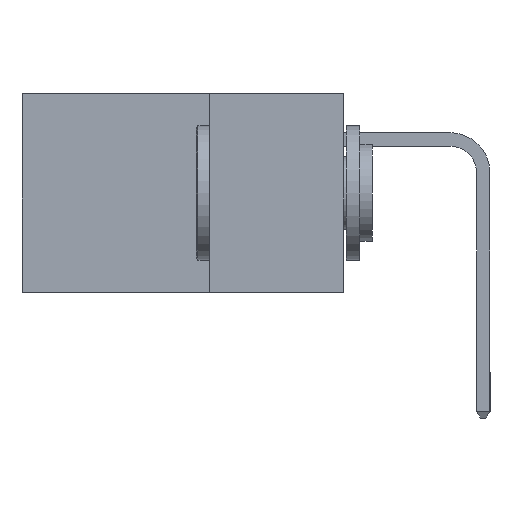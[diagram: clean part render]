
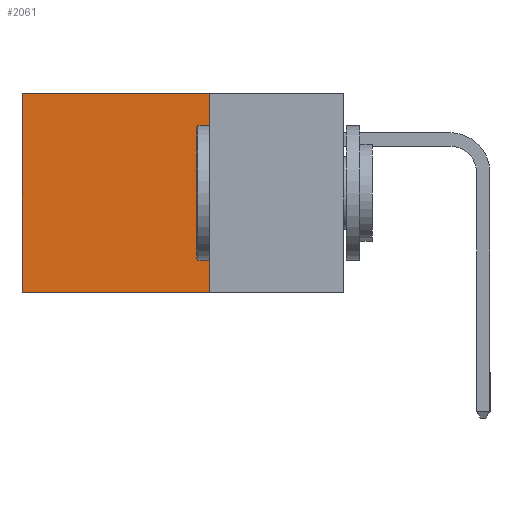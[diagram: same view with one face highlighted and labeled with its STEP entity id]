
A CAD part, left-side view. The second image highlights one B-rep face of the part: STEP entity #2061.
In plain terms, the highlighted planar face has unit normal (-1, 0, 0).
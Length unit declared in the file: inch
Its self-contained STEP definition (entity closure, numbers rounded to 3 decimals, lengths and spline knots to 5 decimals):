
#378 = DIRECTION ( 'NONE',  ( 0., 0., -1. ) ) ;
#1413 = VECTOR ( 'NONE', #378, 39.37008 ) ;
#1704 = CARTESIAN_POINT ( 'NONE',  ( 0.2615, 0.6, -0.37 ) ) ;
#2061 = ADVANCED_FACE ( 'NONE', ( #18170 ), #12680, .F. ) ;
#2657 = VECTOR ( 'NONE', #5814, 39.37008 ) ;
#2699 = LINE ( 'NONE', #21167, #17627 ) ;
#3039 = CARTESIAN_POINT ( 'NONE',  ( 0.2615, 0.25, -0.37 ) ) ;
#4036 = VECTOR ( 'NONE', #19796, 39.37008 ) ;
#5814 = DIRECTION ( 'NONE',  ( 0., 0., -1. ) ) ;
#8389 = DIRECTION ( 'NONE',  ( 0., 1., 0. ) ) ;
#8923 = CARTESIAN_POINT ( 'NONE',  ( 0.2615, 0.25, -0.37 ) ) ;
#9615 = LINE ( 'NONE', #17049, #1413 ) ;
#10564 = CARTESIAN_POINT ( 'NONE',  ( 0.2615, 0.25, 0. ) ) ;
#10827 = ORIENTED_EDGE ( 'NONE', *, *, #17615, .T. ) ;
#10974 = VERTEX_POINT ( 'NONE', #10564 ) ;
#11717 = CARTESIAN_POINT ( 'NONE',  ( 0.2615, 0.25, -0.37 ) ) ;
#11765 = ORIENTED_EDGE ( 'NONE', *, *, #15218, .F. ) ;
#12243 = LINE ( 'NONE', #3039, #4036 ) ;
#12680 = PLANE ( 'NONE',  #15466 ) ;
#12747 = VERTEX_POINT ( 'NONE', #17992 ) ;
#12930 = DIRECTION ( 'NONE',  ( 0., 0., -1. ) ) ;
#15032 = VERTEX_POINT ( 'NONE', #1704 ) ;
#15218 = EDGE_CURVE ( 'NONE', #12747, #15032, #12243, .T. ) ;
#15466 = AXIS2_PLACEMENT_3D ( 'NONE', #8923, #20119, #12930 ) ;
#15508 = LINE ( 'NONE', #11717, #2657 ) ;
#17049 = CARTESIAN_POINT ( 'NONE',  ( 0.2615, 0.6, -0.37 ) ) ;
#17054 = ORIENTED_EDGE ( 'NONE', *, *, #20487, .T. ) ;
#17615 = EDGE_CURVE ( 'NONE', #10974, #20793, #2699, .T. ) ;
#17627 = VECTOR ( 'NONE', #8389, 39.37008 ) ;
#17992 = CARTESIAN_POINT ( 'NONE',  ( 0.2615, 0.25, -0.37 ) ) ;
#18170 = FACE_OUTER_BOUND ( 'NONE', #23583, .T. ) ;
#19796 = DIRECTION ( 'NONE',  ( 0., 1., 0. ) ) ;
#20119 = DIRECTION ( 'NONE',  ( 1., 0., 0. ) ) ;
#20487 = EDGE_CURVE ( 'NONE', #20793, #15032, #9615, .T. ) ;
#20793 = VERTEX_POINT ( 'NONE', #22501 ) ;
#21167 = CARTESIAN_POINT ( 'NONE',  ( 0.2615, 0.25, 0. ) ) ;
#22049 = ORIENTED_EDGE ( 'NONE', *, *, #23962, .F. ) ;
#22501 = CARTESIAN_POINT ( 'NONE',  ( 0.2615, 0.6, 0. ) ) ;
#23583 = EDGE_LOOP ( 'NONE', ( #17054, #11765, #22049, #10827 ) ) ;
#23962 = EDGE_CURVE ( 'NONE', #10974, #12747, #15508, .T. ) ;
